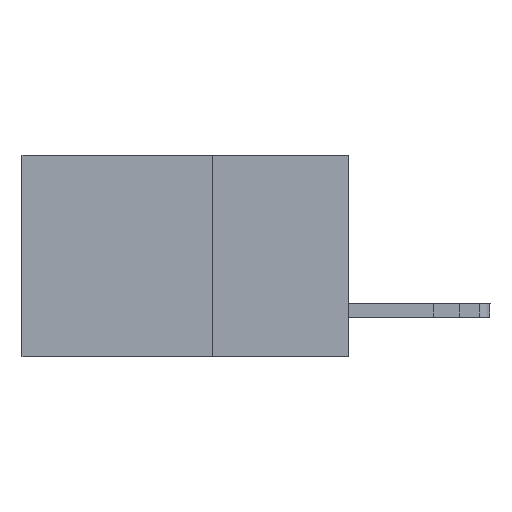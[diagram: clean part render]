
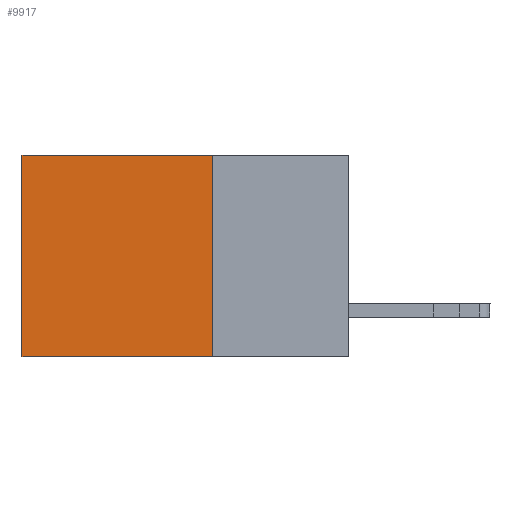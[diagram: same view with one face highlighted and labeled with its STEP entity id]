
A CAD part, left-side view. The second image highlights one B-rep face of the part: STEP entity #9917.
In plain terms, the highlighted planar face has unit normal (-1, 0, 0).
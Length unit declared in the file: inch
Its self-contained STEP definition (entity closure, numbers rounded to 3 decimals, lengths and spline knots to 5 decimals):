
#5 = AXIS2_PLACEMENT_3D ( 'NONE', #9877, #12715, #14252 ) ;
#110 = DIRECTION ( 'NONE',  ( 0., 0., -1. ) ) ;
#1417 = CARTESIAN_POINT ( 'NONE',  ( 0.298, 0.6, -0.37 ) ) ;
#2137 = VECTOR ( 'NONE', #3255, 39.37008 ) ;
#2266 = VERTEX_POINT ( 'NONE', #3459 ) ;
#2551 = CARTESIAN_POINT ( 'NONE',  ( 0.298, 0.25, 0. ) ) ;
#3255 = DIRECTION ( 'NONE',  ( 0., 1., 0. ) ) ;
#3320 = CARTESIAN_POINT ( 'NONE',  ( 0.298, 0.25, 0. ) ) ;
#3459 = CARTESIAN_POINT ( 'NONE',  ( 0.298, 0.6, 0. ) ) ;
#4367 = VERTEX_POINT ( 'NONE', #2551 ) ;
#4691 = CARTESIAN_POINT ( 'NONE',  ( 0.298, 0.6, 0. ) ) ;
#5541 = VECTOR ( 'NONE', #110, 39.37008 ) ;
#8064 = ORIENTED_EDGE ( 'NONE', *, *, #15426, .F. ) ;
#9877 = CARTESIAN_POINT ( 'NONE',  ( 0.298, 0.25, 0. ) ) ;
#9917 = ADVANCED_FACE ( 'NONE', ( #14119 ), #14055, .F. ) ;
#10445 = ORIENTED_EDGE ( 'NONE', *, *, #12889, .T. ) ;
#10531 = CARTESIAN_POINT ( 'NONE',  ( 0.298, 0.25, -0.37 ) ) ;
#11244 = LINE ( 'NONE', #3320, #5541 ) ;
#11630 = VERTEX_POINT ( 'NONE', #1417 ) ;
#12228 = DIRECTION ( 'NONE',  ( 0., 1., 0. ) ) ;
#12715 = DIRECTION ( 'NONE',  ( 1., 0., 0. ) ) ;
#12889 = EDGE_CURVE ( 'NONE', #4367, #2266, #16984, .T. ) ;
#13324 = CARTESIAN_POINT ( 'NONE',  ( 0.298, 0.25, 0. ) ) ;
#13549 = EDGE_CURVE ( 'NONE', #2266, #11630, #13780, .T. ) ;
#13744 = EDGE_CURVE ( 'NONE', #15264, #11630, #18741, .T. ) ;
#13780 = LINE ( 'NONE', #4691, #17390 ) ;
#14055 = PLANE ( 'NONE',  #5 ) ;
#14064 = CARTESIAN_POINT ( 'NONE',  ( 0.298, 0.25, -0.37 ) ) ;
#14119 = FACE_OUTER_BOUND ( 'NONE', #15432, .T. ) ;
#14252 = DIRECTION ( 'NONE',  ( 0., 0., -1. ) ) ;
#15163 = VECTOR ( 'NONE', #12228, 39.37008 ) ;
#15264 = VERTEX_POINT ( 'NONE', #14064 ) ;
#15426 = EDGE_CURVE ( 'NONE', #4367, #15264, #11244, .T. ) ;
#15432 = EDGE_LOOP ( 'NONE', ( #16601, #17901, #8064, #10445 ) ) ;
#16328 = DIRECTION ( 'NONE',  ( 0., 0., -1. ) ) ;
#16601 = ORIENTED_EDGE ( 'NONE', *, *, #13549, .T. ) ;
#16984 = LINE ( 'NONE', #13324, #15163 ) ;
#17390 = VECTOR ( 'NONE', #16328, 39.37008 ) ;
#17901 = ORIENTED_EDGE ( 'NONE', *, *, #13744, .F. ) ;
#18741 = LINE ( 'NONE', #10531, #2137 ) ;
